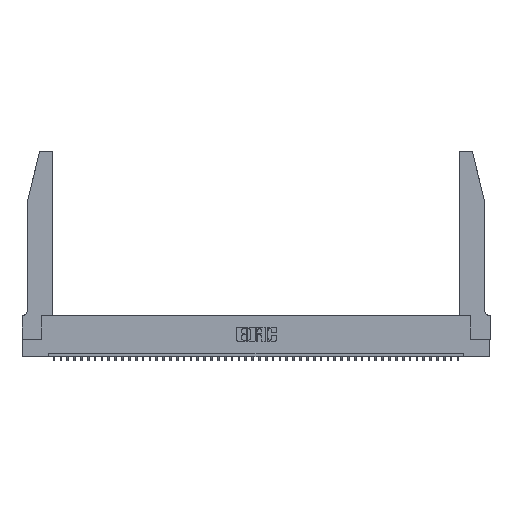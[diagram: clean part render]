
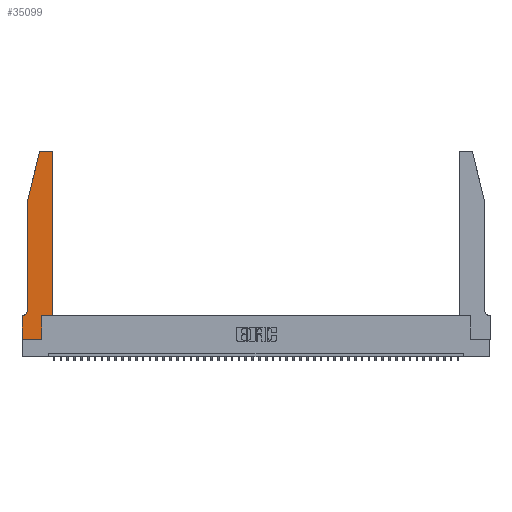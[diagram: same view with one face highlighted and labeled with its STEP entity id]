
A CAD part, top view. The second image highlights one B-rep face of the part: STEP entity #35099.
In plain terms, the highlighted planar face has unit normal (0, 0, 1).
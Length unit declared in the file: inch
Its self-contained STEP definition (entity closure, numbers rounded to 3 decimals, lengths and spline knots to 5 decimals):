
#222 = ORIENTED_EDGE ( 'NONE', *, *, #28000, .T. ) ;
#1317 = CARTESIAN_POINT ( 'NONE',  ( 0.0055, 0.35, 0.37 ) ) ;
#1473 = FACE_OUTER_BOUND ( 'NONE', #22074, .T. ) ;
#1658 = EDGE_CURVE ( 'NONE', #14960, #40271, #26552, .T. ) ;
#3088 = VERTEX_POINT ( 'NONE', #21196 ) ;
#3405 = ORIENTED_EDGE ( 'NONE', *, *, #37552, .T. ) ;
#4547 = DIRECTION ( 'NONE',  ( -0.239, -0.971, 0. ) ) ;
#5162 = EDGE_CURVE ( 'NONE', #20234, #29084, #31437, .T. ) ;
#5216 = CIRCLE ( 'NONE', #5905, 0.03 ) ;
#5905 = AXIS2_PLACEMENT_3D ( 'NONE', #36169, #13460, #31966 ) ;
#5972 = CARTESIAN_POINT ( 'NONE',  ( 0.2865, 0.35, 0.37 ) ) ;
#6119 = CARTESIAN_POINT ( 'NONE',  ( 0., 0., 0.37 ) ) ;
#6699 = DIRECTION ( 'NONE',  ( -1., 0., 0. ) ) ;
#6806 = CARTESIAN_POINT ( 'NONE',  ( 0.4505, 2.72, 0.37 ) ) ;
#7063 = VERTEX_POINT ( 'NONE', #41676 ) ;
#7335 = CIRCLE ( 'NONE', #10808, 0.03 ) ;
#7674 = LINE ( 'NONE', #26794, #31299 ) ;
#8078 = CARTESIAN_POINT ( 'NONE',  ( 0.0755, 2., 0.37 ) ) ;
#8079 = LINE ( 'NONE', #42917, #35712 ) ;
#8949 = CARTESIAN_POINT ( 'NONE',  ( 0., 0.35, 0.37 ) ) ;
#9495 = DIRECTION ( 'NONE',  ( 0., 1., 0. ) ) ;
#9576 = VERTEX_POINT ( 'NONE', #6806 ) ;
#10205 = CARTESIAN_POINT ( 'NONE',  ( 0.0055, 0.42, 0.37 ) ) ;
#10808 = AXIS2_PLACEMENT_3D ( 'NONE', #34816, #12751, #38541 ) ;
#10995 = LINE ( 'NONE', #8078, #39260 ) ;
#11633 = VECTOR ( 'NONE', #9495, 39.37008 ) ;
#11900 = ORIENTED_EDGE ( 'NONE', *, *, #22135, .T. ) ;
#12751 = DIRECTION ( 'NONE',  ( 0., 0., 1. ) ) ;
#13460 = DIRECTION ( 'NONE',  ( 0., 0., 1. ) ) ;
#13804 = EDGE_CURVE ( 'NONE', #35531, #14960, #32258, .T. ) ;
#13963 = CARTESIAN_POINT ( 'NONE',  ( 0.0755, 2., 0.37 ) ) ;
#14577 = EDGE_CURVE ( 'NONE', #40271, #20234, #39858, .T. ) ;
#14960 = VERTEX_POINT ( 'NONE', #46996 ) ;
#15211 = CARTESIAN_POINT ( 'NONE',  ( 0.284, 2.75, 0.37 ) ) ;
#15309 = EDGE_CURVE ( 'NONE', #37199, #18122, #38193, .T. ) ;
#15595 = DIRECTION ( 'NONE',  ( -1., 0., 0. ) ) ;
#16067 = DIRECTION ( 'NONE',  ( 1., 0., 0. ) ) ;
#16166 = VECTOR ( 'NONE', #39142, 39.37008 ) ;
#17269 = CARTESIAN_POINT ( 'NONE',  ( 0.0755, 0.35, 0.37 ) ) ;
#17754 = CARTESIAN_POINT ( 'NONE',  ( 0.4205, 2.75, 0.37 ) ) ;
#18122 = VERTEX_POINT ( 'NONE', #26853 ) ;
#18495 = LINE ( 'NONE', #44528, #43822 ) ;
#19928 = DIRECTION ( 'NONE',  ( 0., 0., 1. ) ) ;
#20133 = DIRECTION ( 'NONE',  ( 0., -1., 0. ) ) ;
#20234 = VERTEX_POINT ( 'NONE', #36013 ) ;
#20541 = CARTESIAN_POINT ( 'NONE',  ( 0.0755, 2., 0.37 ) ) ;
#21196 = CARTESIAN_POINT ( 'NONE',  ( 0.4505, 0.35, 0.37 ) ) ;
#22074 = EDGE_LOOP ( 'NONE', ( #30499, #28511, #40588, #43975, #26674, #35205, #32904, #222, #40363, #43791, #11900, #3405 ) ) ;
#22135 = EDGE_CURVE ( 'NONE', #3088, #9576, #35978, .T. ) ;
#22790 = VECTOR ( 'NONE', #20133, 39.37008 ) ;
#23819 = EDGE_CURVE ( 'NONE', #7063, #35531, #10995, .T. ) ;
#26046 = EDGE_CURVE ( 'NONE', #43402, #7063, #7335, .T. ) ;
#26552 = CIRCLE ( 'NONE', #33093, 0.07 ) ;
#26674 = ORIENTED_EDGE ( 'NONE', *, *, #1658, .T. ) ;
#26794 = CARTESIAN_POINT ( 'NONE',  ( 0., 0., 0.37 ) ) ;
#26853 = CARTESIAN_POINT ( 'NONE',  ( 0.2865, 0.35, 0.37 ) ) ;
#27618 = VERTEX_POINT ( 'NONE', #17754 ) ;
#28000 = EDGE_CURVE ( 'NONE', #29084, #37199, #7674, .T. ) ;
#28511 = ORIENTED_EDGE ( 'NONE', *, *, #26046, .T. ) ;
#29084 = VERTEX_POINT ( 'NONE', #6119 ) ;
#30499 = ORIENTED_EDGE ( 'NONE', *, *, #44827, .T. ) ;
#30824 = PLANE ( 'NONE',  #40386 ) ;
#31299 = VECTOR ( 'NONE', #33804, 39.37008 ) ;
#31437 = LINE ( 'NONE', #45523, #22790 ) ;
#31966 = DIRECTION ( 'NONE',  ( 1., 0., 0. ) ) ;
#32258 = LINE ( 'NONE', #13963, #40899 ) ;
#32904 = ORIENTED_EDGE ( 'NONE', *, *, #5162, .T. ) ;
#33093 = AXIS2_PLACEMENT_3D ( 'NONE', #10205, #35998, #6699 ) ;
#33804 = DIRECTION ( 'NONE',  ( 1., 0., 0. ) ) ;
#34816 = CARTESIAN_POINT ( 'NONE',  ( 0.284, 2.72, 0.37 ) ) ;
#35099 = ADVANCED_FACE ( 'NONE', ( #1473 ), #30824, .T. ) ;
#35205 = ORIENTED_EDGE ( 'NONE', *, *, #14577, .T. ) ;
#35531 = VERTEX_POINT ( 'NONE', #20541 ) ;
#35712 = VECTOR ( 'NONE', #42266, 39.37008 ) ;
#35978 = LINE ( 'NONE', #43893, #43987 ) ;
#35998 = DIRECTION ( 'NONE',  ( 0., 0., -1. ) ) ;
#36013 = CARTESIAN_POINT ( 'NONE',  ( 0., 0.35, 0.37 ) ) ;
#36169 = CARTESIAN_POINT ( 'NONE',  ( 0.4205, 2.72, 0.37 ) ) ;
#37199 = VERTEX_POINT ( 'NONE', #42456 ) ;
#37552 = EDGE_CURVE ( 'NONE', #9576, #27618, #5216, .T. ) ;
#38193 = LINE ( 'NONE', #5972, #11633 ) ;
#38541 = DIRECTION ( 'NONE',  ( 1., 0., 0. ) ) ;
#39142 = DIRECTION ( 'NONE',  ( -1., 0., 0. ) ) ;
#39260 = VECTOR ( 'NONE', #4547, 39.37008 ) ;
#39420 = DIRECTION ( 'NONE',  ( 0., -1., 0. ) ) ;
#39858 = LINE ( 'NONE', #17269, #16166 ) ;
#40271 = VERTEX_POINT ( 'NONE', #1317 ) ;
#40363 = ORIENTED_EDGE ( 'NONE', *, *, #15309, .T. ) ;
#40386 = AXIS2_PLACEMENT_3D ( 'NONE', #8949, #19928, #16067 ) ;
#40588 = ORIENTED_EDGE ( 'NONE', *, *, #23819, .T. ) ;
#40899 = VECTOR ( 'NONE', #39420, 39.37008 ) ;
#41676 = CARTESIAN_POINT ( 'NONE',  ( 0.25487, 2.72718, 0.37 ) ) ;
#42266 = DIRECTION ( 'NONE',  ( 1., 0., 0. ) ) ;
#42456 = CARTESIAN_POINT ( 'NONE',  ( 0.2865, 0., 0.37 ) ) ;
#42917 = CARTESIAN_POINT ( 'NONE',  ( 0.4505, 0.35, 0.37 ) ) ;
#43402 = VERTEX_POINT ( 'NONE', #15211 ) ;
#43791 = ORIENTED_EDGE ( 'NONE', *, *, #45133, .T. ) ;
#43822 = VECTOR ( 'NONE', #15595, 39.37008 ) ;
#43893 = CARTESIAN_POINT ( 'NONE',  ( 0.4505, 0.35, 0.37 ) ) ;
#43975 = ORIENTED_EDGE ( 'NONE', *, *, #13804, .T. ) ;
#43987 = VECTOR ( 'NONE', #47579, 39.37008 ) ;
#44528 = CARTESIAN_POINT ( 'NONE',  ( 0.2605, 2.75, 0.37 ) ) ;
#44827 = EDGE_CURVE ( 'NONE', #27618, #43402, #18495, .T. ) ;
#45133 = EDGE_CURVE ( 'NONE', #18122, #3088, #8079, .T. ) ;
#45523 = CARTESIAN_POINT ( 'NONE',  ( 0., 0., 0.37 ) ) ;
#46996 = CARTESIAN_POINT ( 'NONE',  ( 0.0755, 0.42, 0.37 ) ) ;
#47579 = DIRECTION ( 'NONE',  ( 0., 1., 0. ) ) ;
